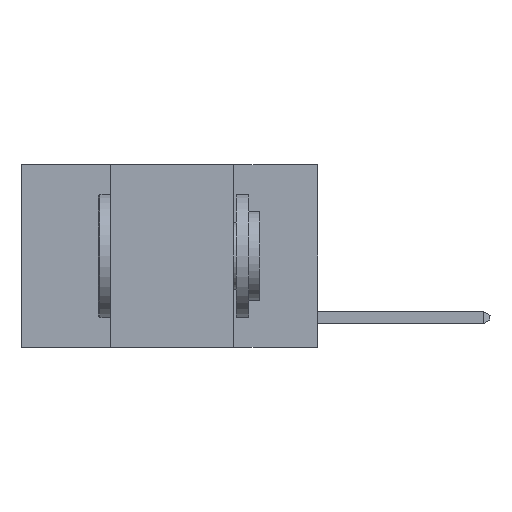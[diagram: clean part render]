
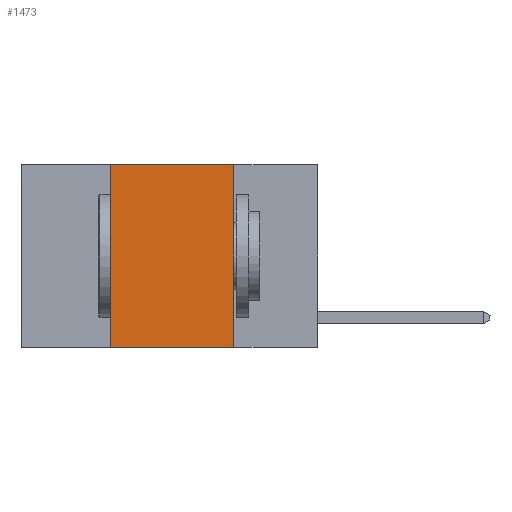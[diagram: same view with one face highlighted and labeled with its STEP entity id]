
A CAD part, left-side view. The second image highlights one B-rep face of the part: STEP entity #1473.
In plain terms, the highlighted planar face has unit normal (-1, 0, 0).
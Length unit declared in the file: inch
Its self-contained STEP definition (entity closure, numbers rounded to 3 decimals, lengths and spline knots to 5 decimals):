
#264 = ORIENTED_EDGE ( 'NONE', *, *, #10965, .F. ) ;
#622 = CARTESIAN_POINT ( 'NONE',  ( 0., 0.17, 0. ) ) ;
#992 = VECTOR ( 'NONE', #8913, 39.37008 ) ;
#1131 = EDGE_LOOP ( 'NONE', ( #10217, #264, #9751, #1689 ) ) ;
#1138 = CARTESIAN_POINT ( 'NONE',  ( 0., 0.42, 0. ) ) ;
#1473 = ADVANCED_FACE ( 'NONE', ( #10881 ), #3219, .F. ) ;
#1689 = ORIENTED_EDGE ( 'NONE', *, *, #8460, .T. ) ;
#2498 = LINE ( 'NONE', #622, #992 ) ;
#3219 = PLANE ( 'NONE',  #6757 ) ;
#3557 = CARTESIAN_POINT ( 'NONE',  ( 0., 0.17, 0. ) ) ;
#3974 = CARTESIAN_POINT ( 'NONE',  ( 0., 0.17, -0.37 ) ) ;
#4376 = LINE ( 'NONE', #9120, #8960 ) ;
#4436 = CARTESIAN_POINT ( 'NONE',  ( 0., 0.42, -0.37 ) ) ;
#4896 = EDGE_CURVE ( 'NONE', #8540, #12046, #7683, .T. ) ;
#6757 = AXIS2_PLACEMENT_3D ( 'NONE', #10761, #11751, #9806 ) ;
#6866 = CARTESIAN_POINT ( 'NONE',  ( 0., 0.42, 0. ) ) ;
#7490 = DIRECTION ( 'NONE',  ( 0., -1., 0. ) ) ;
#7683 = LINE ( 'NONE', #1138, #11454 ) ;
#8429 = LINE ( 'NONE', #9097, #11397 ) ;
#8460 = EDGE_CURVE ( 'NONE', #8540, #9216, #4376, .T. ) ;
#8540 = VERTEX_POINT ( 'NONE', #4436 ) ;
#8764 = DIRECTION ( 'NONE',  ( 0., 0., 1. ) ) ;
#8913 = DIRECTION ( 'NONE',  ( 0., 0., -1. ) ) ;
#8960 = VECTOR ( 'NONE', #11108, 39.37008 ) ;
#9097 = CARTESIAN_POINT ( 'NONE',  ( 0., 0.6, 0. ) ) ;
#9120 = CARTESIAN_POINT ( 'NONE',  ( 0., 0.6, -0.37 ) ) ;
#9216 = VERTEX_POINT ( 'NONE', #3974 ) ;
#9721 = EDGE_CURVE ( 'NONE', #11265, #9216, #2498, .T. ) ;
#9751 = ORIENTED_EDGE ( 'NONE', *, *, #4896, .F. ) ;
#9806 = DIRECTION ( 'NONE',  ( 0., 0., -1. ) ) ;
#10217 = ORIENTED_EDGE ( 'NONE', *, *, #9721, .F. ) ;
#10761 = CARTESIAN_POINT ( 'NONE',  ( 0., 0.6, 0. ) ) ;
#10881 = FACE_OUTER_BOUND ( 'NONE', #1131, .T. ) ;
#10965 = EDGE_CURVE ( 'NONE', #12046, #11265, #8429, .T. ) ;
#11108 = DIRECTION ( 'NONE',  ( 0., -1., 0. ) ) ;
#11265 = VERTEX_POINT ( 'NONE', #3557 ) ;
#11397 = VECTOR ( 'NONE', #7490, 39.37008 ) ;
#11454 = VECTOR ( 'NONE', #8764, 39.37008 ) ;
#11751 = DIRECTION ( 'NONE',  ( 1., 0., 0. ) ) ;
#12046 = VERTEX_POINT ( 'NONE', #6866 ) ;
